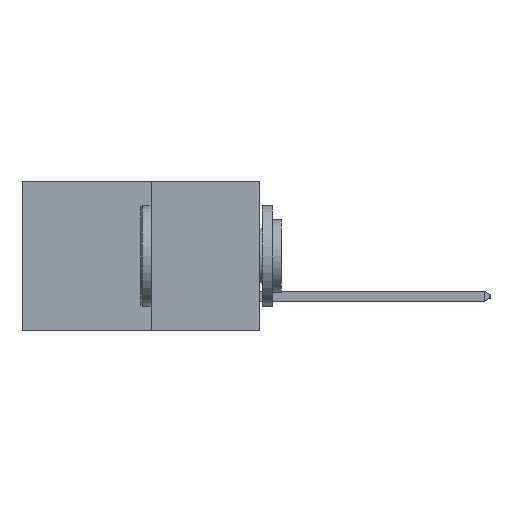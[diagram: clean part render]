
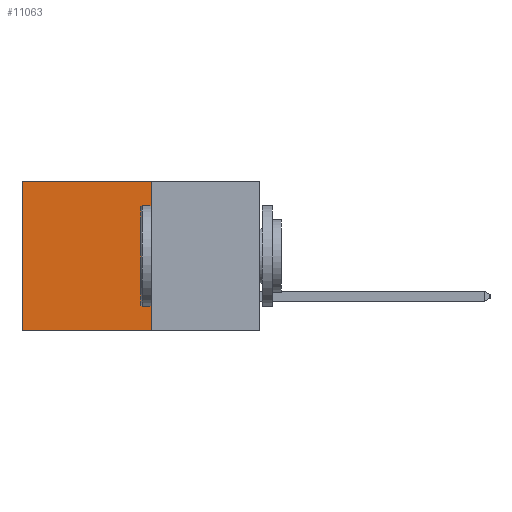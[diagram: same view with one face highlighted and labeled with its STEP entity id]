
A CAD part, left-side view. The second image highlights one B-rep face of the part: STEP entity #11063.
In plain terms, the highlighted planar face has unit normal (-1, 0, 0).
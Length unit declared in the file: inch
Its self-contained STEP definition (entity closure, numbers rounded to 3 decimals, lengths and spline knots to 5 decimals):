
#349 = VECTOR ( 'NONE', #4274, 39.37008 ) ;
#480 = LINE ( 'NONE', #6460, #1090 ) ;
#559 = EDGE_CURVE ( 'NONE', #4536, #8076, #3123, .T. ) ;
#818 = ORIENTED_EDGE ( 'NONE', *, *, #1863, .T. ) ;
#1012 = EDGE_CURVE ( 'NONE', #8076, #10976, #10949, .T. ) ;
#1090 = VECTOR ( 'NONE', #5961, 39.37008 ) ;
#1399 = CARTESIAN_POINT ( 'NONE',  ( 0.277, 0.59, -0.37 ) ) ;
#1863 = EDGE_CURVE ( 'NONE', #4536, #11142, #8861, .T. ) ;
#1864 = CARTESIAN_POINT ( 'NONE',  ( 0.277, 0.27, 0. ) ) ;
#1918 = DIRECTION ( 'NONE',  ( 0., 1., 0. ) ) ;
#2787 = CARTESIAN_POINT ( 'NONE',  ( 0.277, 0.27, -0.37 ) ) ;
#2958 = ORIENTED_EDGE ( 'NONE', *, *, #3772, .T. ) ;
#3123 = LINE ( 'NONE', #4351, #349 ) ;
#3338 = DIRECTION ( 'NONE',  ( 1., 0., 0. ) ) ;
#3772 = EDGE_CURVE ( 'NONE', #11142, #10976, #480, .T. ) ;
#4274 = DIRECTION ( 'NONE',  ( 0., 0., -1. ) ) ;
#4351 = CARTESIAN_POINT ( 'NONE',  ( 0.277, 0.27, -0.37 ) ) ;
#4536 = VERTEX_POINT ( 'NONE', #6882 ) ;
#4645 = AXIS2_PLACEMENT_3D ( 'NONE', #7040, #3338, #9718 ) ;
#5961 = DIRECTION ( 'NONE',  ( 0., 0., -1. ) ) ;
#6460 = CARTESIAN_POINT ( 'NONE',  ( 0.277, 0.59, -0.37 ) ) ;
#6882 = CARTESIAN_POINT ( 'NONE',  ( 0.277, 0.27, 0. ) ) ;
#7040 = CARTESIAN_POINT ( 'NONE',  ( 0.277, 0.27, -0.37 ) ) ;
#7294 = DIRECTION ( 'NONE',  ( 0., 1., 0. ) ) ;
#7618 = FACE_OUTER_BOUND ( 'NONE', #7689, .T. ) ;
#7689 = EDGE_LOOP ( 'NONE', ( #2958, #7876, #10230, #818 ) ) ;
#7851 = CARTESIAN_POINT ( 'NONE',  ( 0.277, 0.27, -0.37 ) ) ;
#7876 = ORIENTED_EDGE ( 'NONE', *, *, #1012, .F. ) ;
#8076 = VERTEX_POINT ( 'NONE', #7851 ) ;
#8614 = VECTOR ( 'NONE', #1918, 39.37008 ) ;
#8826 = PLANE ( 'NONE',  #4645 ) ;
#8861 = LINE ( 'NONE', #1864, #10927 ) ;
#9718 = DIRECTION ( 'NONE',  ( 0., 0., -1. ) ) ;
#10230 = ORIENTED_EDGE ( 'NONE', *, *, #559, .F. ) ;
#10683 = CARTESIAN_POINT ( 'NONE',  ( 0.277, 0.59, 0. ) ) ;
#10927 = VECTOR ( 'NONE', #7294, 39.37008 ) ;
#10949 = LINE ( 'NONE', #2787, #8614 ) ;
#10976 = VERTEX_POINT ( 'NONE', #1399 ) ;
#11063 = ADVANCED_FACE ( 'NONE', ( #7618 ), #8826, .F. ) ;
#11142 = VERTEX_POINT ( 'NONE', #10683 ) ;
